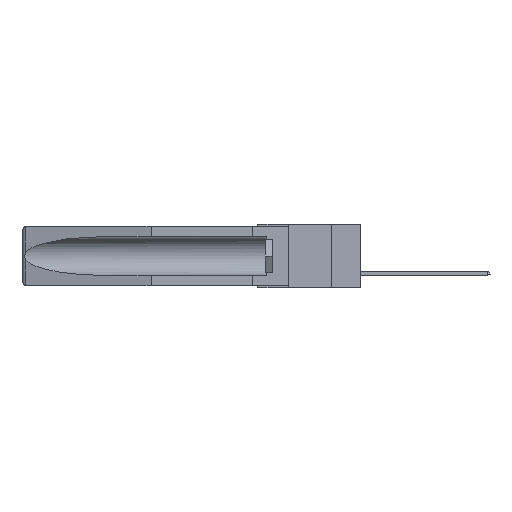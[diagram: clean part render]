
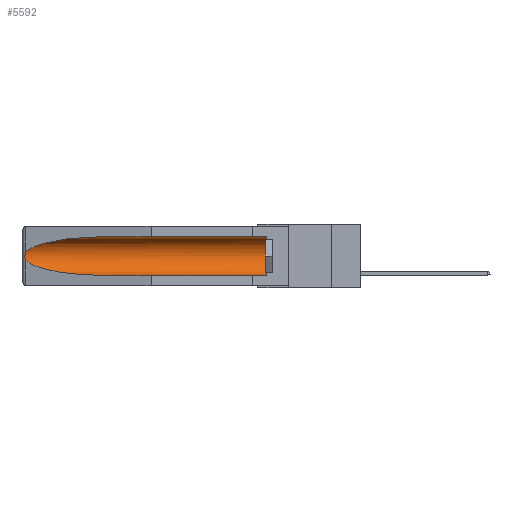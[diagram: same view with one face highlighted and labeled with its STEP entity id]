
A CAD part, left-side view. The second image highlights one B-rep face of the part: STEP entity #5592.
In plain terms, the highlighted cylindrical face has radius 2.857 mm (diameter 5.715 mm), a partial arc.
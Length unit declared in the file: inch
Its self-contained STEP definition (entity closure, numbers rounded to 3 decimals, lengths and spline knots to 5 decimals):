
#209 = DIRECTION ( 'NONE',  ( 0., -1., 0. ) ) ;
#345 =( BOUNDED_CURVE ( )  B_SPLINE_CURVE ( 3, ( #16953, #4129, #5591, #8814 ),
 .UNSPECIFIED., .F., .F. ) 
 B_SPLINE_CURVE_WITH_KNOTS ( ( 4, 4 ),
 ( 4.71239, 6.08839 ),
 .UNSPECIFIED. ) 
 CURVE ( )  GEOMETRIC_REPRESENTATION_ITEM ( )  RATIONAL_B_SPLINE_CURVE ( ( 1., 0.848, 0.848, 1. ) ) 
 REPRESENTATION_ITEM ( '' )  );
#1532 = CARTESIAN_POINT ( 'NONE',  ( 0.155, 1.07973, -0.284 ) ) ;
#1768 = VERTEX_POINT ( 'NONE', #1777 ) ;
#1777 = CARTESIAN_POINT ( 'NONE',  ( 0.155, 0.126, -0.059 ) ) ;
#1874 = VERTEX_POINT ( 'NONE', #14304 ) ;
#3004 = CARTESIAN_POINT ( 'NONE',  ( 0.21114, 1.30732, -0.284 ) ) ;
#3203 = CIRCLE ( 'NONE', #13228, 0.1125 ) ;
#3535 = DIRECTION ( 'NONE',  ( 0., 0., 1. ) ) ;
#4075 = ORIENTED_EDGE ( 'NONE', *, *, #17763, .T. ) ;
#4129 = CARTESIAN_POINT ( 'NONE',  ( 0.21114, 1.30732, -0.059 ) ) ;
#4188 = CARTESIAN_POINT ( 'NONE',  ( 0.26537, 1.52718, -0.19328 ) ) ;
#5331 = ORIENTED_EDGE ( 'NONE', *, *, #11149, .F. ) ;
#5591 = CARTESIAN_POINT ( 'NONE',  ( 0.25451, 1.48313, -0.09465 ) ) ;
#5592 = ADVANCED_FACE ( 'NONE', ( #16508 ), #16774, .F. ) ;
#5724 = CARTESIAN_POINT ( 'NONE',  ( 0.26655, 1.53094, -0.18657 ) ) ;
#5933 = VERTEX_POINT ( 'NONE', #18613 ) ;
#6024 = CARTESIAN_POINT ( 'NONE',  ( 0.26597, 1.52961, -0.15275 ) ) ;
#6291 = VECTOR ( 'NONE', #12099, 39.37008 ) ;
#6419 = CARTESIAN_POINT ( 'NONE',  ( 0.2673, 1.5327, -0.16383 ) ) ;
#6826 = CARTESIAN_POINT ( 'NONE',  ( 0.2675, 1.53308, -0.16763 ) ) ;
#7114 = CARTESIAN_POINT ( 'NONE',  ( 0.26597, 1.5296, -0.19026 ) ) ;
#7610 = ORIENTED_EDGE ( 'NONE', *, *, #17948, .T. ) ;
#7899 = CARTESIAN_POINT ( 'NONE',  ( 0.25451, 1.48313, -0.24835 ) ) ;
#8057 = LINE ( 'NONE', #16909, #8304 ) ;
#8304 = VECTOR ( 'NONE', #15265, 39.37008 ) ;
#8373 = VERTEX_POINT ( 'NONE', #1532 ) ;
#8814 = CARTESIAN_POINT ( 'NONE',  ( 0.26537, 1.52718, -0.14972 ) ) ;
#9453 = CARTESIAN_POINT ( 'NONE',  ( 0.155, -0.30754, -0.284 ) ) ;
#9903 = CARTESIAN_POINT ( 'NONE',  ( 0.155, 0.126, -0.1715 ) ) ;
#10988 = VERTEX_POINT ( 'NONE', #13629 ) ;
#11008 = EDGE_CURVE ( 'NONE', #1768, #1874, #8057, .T. ) ;
#11149 = EDGE_CURVE ( 'NONE', #10988, #8373, #19689, .T. ) ;
#11991 = ORIENTED_EDGE ( 'NONE', *, *, #11008, .T. ) ;
#12099 = DIRECTION ( 'NONE',  ( 0., 1., 0. ) ) ;
#12442 = AXIS2_PLACEMENT_3D ( 'NONE', #15551, #17189, #15414 ) ;
#12894 = CARTESIAN_POINT ( 'NONE',  ( 0.26654, 1.53092, -0.15636 ) ) ;
#13047 = CARTESIAN_POINT ( 'NONE',  ( 0.26537, 1.52718, -0.14972 ) ) ;
#13228 = AXIS2_PLACEMENT_3D ( 'NONE', #9903, #209, #3535 ) ;
#13377 =( BOUNDED_CURVE ( )  B_SPLINE_CURVE ( 3, ( #20765, #7899, #3004, #14368 ),
 .UNSPECIFIED., .F., .F. ) 
 B_SPLINE_CURVE_WITH_KNOTS ( ( 4, 4 ),
 ( 0.1948, 1.5708 ),
 .UNSPECIFIED. ) 
 CURVE ( )  GEOMETRIC_REPRESENTATION_ITEM ( )  RATIONAL_B_SPLINE_CURVE ( ( 1., 0.848, 0.848, 1. ) ) 
 REPRESENTATION_ITEM ( '' )  );
#13629 = CARTESIAN_POINT ( 'NONE',  ( 0.155, 0.126, -0.284 ) ) ;
#14192 = VERTEX_POINT ( 'NONE', #13047 ) ;
#14304 = CARTESIAN_POINT ( 'NONE',  ( 0.155, 1.07973, -0.059 ) ) ;
#14368 = CARTESIAN_POINT ( 'NONE',  ( 0.155, 1.07973, -0.284 ) ) ;
#14721 = B_SPLINE_CURVE_WITH_KNOTS ( 'NONE', 3,
 ( #15671, #6024, #12894, #6419, #6826, #16632, #19878, #5724, #7114, #4188 ),
 .UNSPECIFIED., .F., .F.,
 ( 4, 2, 2, 2, 4 ),
 ( 0., 0.00029, 0.00058, 0.00087, 0.00117 ),
 .UNSPECIFIED. ) ;
#15265 = DIRECTION ( 'NONE',  ( 0., 1., 0. ) ) ;
#15414 = DIRECTION ( 'NONE',  ( 0., 0., 1. ) ) ;
#15551 = CARTESIAN_POINT ( 'NONE',  ( 0.155, -0.30754, -0.1715 ) ) ;
#15671 = CARTESIAN_POINT ( 'NONE',  ( 0.26537, 1.52718, -0.14972 ) ) ;
#15815 = EDGE_LOOP ( 'NONE', ( #4075, #7610, #20387, #5331, #16467, #11991 ) ) ;
#16467 = ORIENTED_EDGE ( 'NONE', *, *, #16525, .T. ) ;
#16508 = FACE_OUTER_BOUND ( 'NONE', #15815, .T. ) ;
#16525 = EDGE_CURVE ( 'NONE', #10988, #1768, #3203, .T. ) ;
#16632 = CARTESIAN_POINT ( 'NONE',  ( 0.2675, 1.53308, -0.17534 ) ) ;
#16774 = CYLINDRICAL_SURFACE ( 'NONE', #12442, 0.1125 ) ;
#16909 = CARTESIAN_POINT ( 'NONE',  ( 0.155, -0.30754, -0.059 ) ) ;
#16953 = CARTESIAN_POINT ( 'NONE',  ( 0.155, 1.07973, -0.059 ) ) ;
#17116 = EDGE_CURVE ( 'NONE', #5933, #8373, #13377, .T. ) ;
#17189 = DIRECTION ( 'NONE',  ( 0., 1., 0. ) ) ;
#17763 = EDGE_CURVE ( 'NONE', #1874, #14192, #345, .T. ) ;
#17948 = EDGE_CURVE ( 'NONE', #14192, #5933, #14721, .T. ) ;
#18613 = CARTESIAN_POINT ( 'NONE',  ( 0.26537, 1.52718, -0.19328 ) ) ;
#19689 = LINE ( 'NONE', #9453, #6291 ) ;
#19878 = CARTESIAN_POINT ( 'NONE',  ( 0.2673, 1.53269, -0.17917 ) ) ;
#20387 = ORIENTED_EDGE ( 'NONE', *, *, #17116, .T. ) ;
#20765 = CARTESIAN_POINT ( 'NONE',  ( 0.26537, 1.52718, -0.19328 ) ) ;
